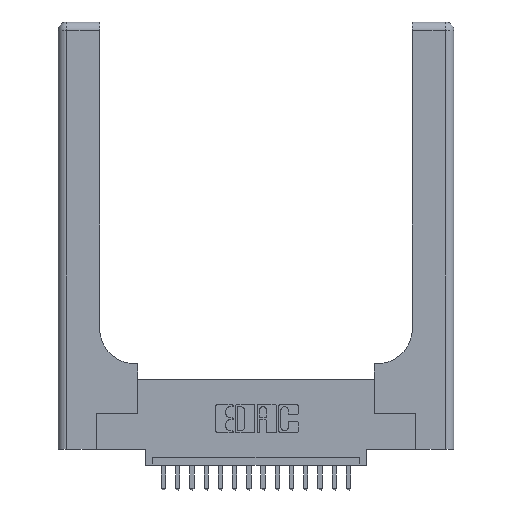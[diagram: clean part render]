
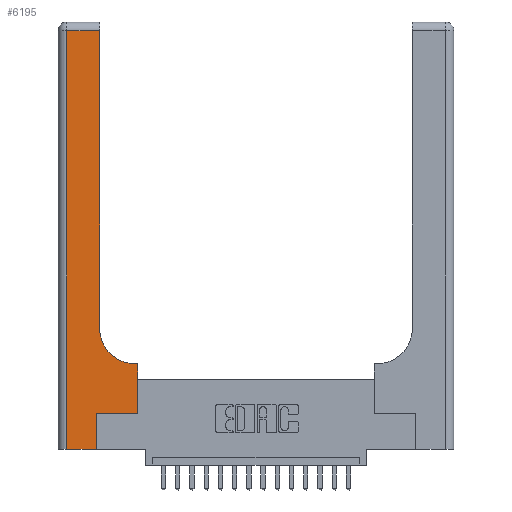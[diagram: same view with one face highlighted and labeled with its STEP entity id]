
A CAD part, top view. The second image highlights one B-rep face of the part: STEP entity #6195.
In plain terms, the highlighted planar face has unit normal (0, 0, 1).
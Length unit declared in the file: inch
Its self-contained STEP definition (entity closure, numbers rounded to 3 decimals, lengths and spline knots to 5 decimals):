
#48 = CARTESIAN_POINT ( 'NONE',  ( 0.5585, 0.6, 0.37 ) ) ;
#52 = CARTESIAN_POINT ( 'NONE',  ( 0., 3., 0.37 ) ) ;
#325 = EDGE_CURVE ( 'NONE', #15766, #13900, #18943, .T. ) ;
#832 = VECTOR ( 'NONE', #4143, 39.37008 ) ;
#1177 = EDGE_CURVE ( 'NONE', #13900, #14585, #15948, .T. ) ;
#1362 = FACE_OUTER_BOUND ( 'NONE', #18230, .T. ) ;
#1371 = DIRECTION ( 'NONE',  ( -1., 0., 0. ) ) ;
#1585 = CARTESIAN_POINT ( 'NONE',  ( 0.269, 0.25, 0.37 ) ) ;
#1635 = DIRECTION ( 'NONE',  ( -1., 0., 0. ) ) ;
#1694 = CARTESIAN_POINT ( 'NONE',  ( 0., 0., 0.37 ) ) ;
#2590 = ORIENTED_EDGE ( 'NONE', *, *, #15834, .T. ) ;
#3167 = CARTESIAN_POINT ( 'NONE',  ( 0.269, 0., 0.37 ) ) ;
#3985 = VERTEX_POINT ( 'NONE', #12323 ) ;
#4142 = CARTESIAN_POINT ( 'NONE',  ( 0.5585, 0.25, 0.37 ) ) ;
#4143 = DIRECTION ( 'NONE',  ( 0., 1., 0. ) ) ;
#4580 = CARTESIAN_POINT ( 'NONE',  ( 0., 2.94, 0.37 ) ) ;
#4636 = CARTESIAN_POINT ( 'NONE',  ( 0.2915, 0.6, 0.37 ) ) ;
#4918 = EDGE_CURVE ( 'NONE', #3985, #17916, #9988, .T. ) ;
#4936 = VECTOR ( 'NONE', #7543, 39.37008 ) ;
#5139 = VERTEX_POINT ( 'NONE', #12796 ) ;
#5212 = CARTESIAN_POINT ( 'NONE',  ( 0.2915, 2.94, 0.37 ) ) ;
#5394 = VECTOR ( 'NONE', #11621, 39.37008 ) ;
#5434 = ORIENTED_EDGE ( 'NONE', *, *, #4918, .T. ) ;
#5975 = DIRECTION ( 'NONE',  ( 0., 0., -1. ) ) ;
#6195 = ADVANCED_FACE ( 'NONE', ( #1362 ), #12128, .F. ) ;
#6277 = DIRECTION ( 'NONE',  ( 0., 1., 0. ) ) ;
#6708 = LINE ( 'NONE', #1694, #16249 ) ;
#7543 = DIRECTION ( 'NONE',  ( 0., -1., 0. ) ) ;
#7789 = EDGE_CURVE ( 'NONE', #13838, #3985, #19189, .T. ) ;
#7906 = CARTESIAN_POINT ( 'NONE',  ( 0.06, 3., 0.37 ) ) ;
#8530 = CARTESIAN_POINT ( 'NONE',  ( 0.269, 0., 0.37 ) ) ;
#8716 = DIRECTION ( 'NONE',  ( -1., 0., 0. ) ) ;
#9070 = VERTEX_POINT ( 'NONE', #11427 ) ;
#9212 = VECTOR ( 'NONE', #17917, 39.37008 ) ;
#9568 = VECTOR ( 'NONE', #6277, 39.37008 ) ;
#9592 = VECTOR ( 'NONE', #8716, 39.37008 ) ;
#9988 = CIRCLE ( 'NONE', #10682, 0.25 ) ;
#10120 = CARTESIAN_POINT ( 'NONE',  ( 0.2915, 3., 0.37 ) ) ;
#10486 = ORIENTED_EDGE ( 'NONE', *, *, #18361, .T. ) ;
#10682 = AXIS2_PLACEMENT_3D ( 'NONE', #15671, #17420, #15937 ) ;
#11100 = VECTOR ( 'NONE', #1635, 39.37008 ) ;
#11287 = LINE ( 'NONE', #4580, #9592 ) ;
#11427 = CARTESIAN_POINT ( 'NONE',  ( 0.06, 2.94, 0.37 ) ) ;
#11620 = EDGE_CURVE ( 'NONE', #17916, #16001, #16845, .T. ) ;
#11621 = DIRECTION ( 'NONE',  ( 0., 1., 0. ) ) ;
#12128 = PLANE ( 'NONE',  #19748 ) ;
#12209 = ORIENTED_EDGE ( 'NONE', *, *, #14304, .T. ) ;
#12323 = CARTESIAN_POINT ( 'NONE',  ( 0.5415, 0.6, 0.37 ) ) ;
#12796 = CARTESIAN_POINT ( 'NONE',  ( 0.06, 0., 0.37 ) ) ;
#13026 = LINE ( 'NONE', #7906, #4936 ) ;
#13097 = ORIENTED_EDGE ( 'NONE', *, *, #11620, .T. ) ;
#13838 = VERTEX_POINT ( 'NONE', #48 ) ;
#13900 = VERTEX_POINT ( 'NONE', #1585 ) ;
#13921 = CARTESIAN_POINT ( 'NONE',  ( 0.2915, 0.85, 0.37 ) ) ;
#14304 = EDGE_CURVE ( 'NONE', #16001, #9070, #11287, .T. ) ;
#14585 = VERTEX_POINT ( 'NONE', #4142 ) ;
#15534 = DIRECTION ( 'NONE',  ( 1., 0., 0. ) ) ;
#15671 = CARTESIAN_POINT ( 'NONE',  ( 0.5415, 0.85, 0.37 ) ) ;
#15766 = VERTEX_POINT ( 'NONE', #3167 ) ;
#15834 = EDGE_CURVE ( 'NONE', #14585, #13838, #17924, .T. ) ;
#15880 = EDGE_CURVE ( 'NONE', #5139, #15766, #6708, .T. ) ;
#15937 = DIRECTION ( 'NONE',  ( 1., 0., 0. ) ) ;
#15948 = LINE ( 'NONE', #16453, #9212 ) ;
#16001 = VERTEX_POINT ( 'NONE', #5212 ) ;
#16249 = VECTOR ( 'NONE', #15534, 39.37008 ) ;
#16359 = ORIENTED_EDGE ( 'NONE', *, *, #1177, .T. ) ;
#16453 = CARTESIAN_POINT ( 'NONE',  ( 0.269, 0.25, 0.37 ) ) ;
#16641 = ORIENTED_EDGE ( 'NONE', *, *, #15880, .T. ) ;
#16698 = CARTESIAN_POINT ( 'NONE',  ( 0.5585, 0.25, 0.37 ) ) ;
#16845 = LINE ( 'NONE', #10120, #5394 ) ;
#17063 = ORIENTED_EDGE ( 'NONE', *, *, #325, .T. ) ;
#17420 = DIRECTION ( 'NONE',  ( 0., 0., -1. ) ) ;
#17916 = VERTEX_POINT ( 'NONE', #13921 ) ;
#17917 = DIRECTION ( 'NONE',  ( 1., 0., 0. ) ) ;
#17924 = LINE ( 'NONE', #16698, #9568 ) ;
#18230 = EDGE_LOOP ( 'NONE', ( #13097, #12209, #10486, #16641, #17063, #16359, #2590, #18504, #5434 ) ) ;
#18361 = EDGE_CURVE ( 'NONE', #9070, #5139, #13026, .T. ) ;
#18504 = ORIENTED_EDGE ( 'NONE', *, *, #7789, .T. ) ;
#18943 = LINE ( 'NONE', #8530, #832 ) ;
#19189 = LINE ( 'NONE', #4636, #11100 ) ;
#19748 = AXIS2_PLACEMENT_3D ( 'NONE', #52, #5975, #1371 ) ;
